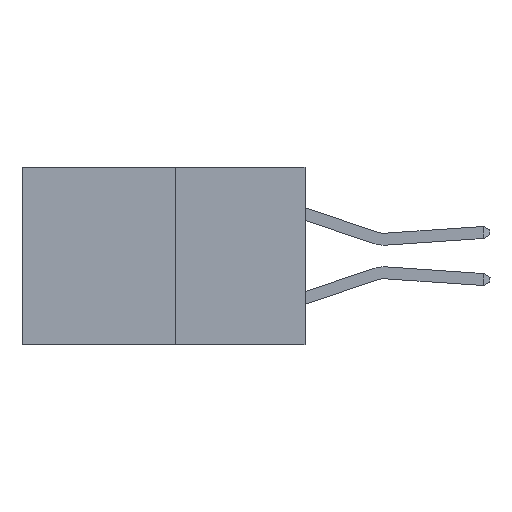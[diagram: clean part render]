
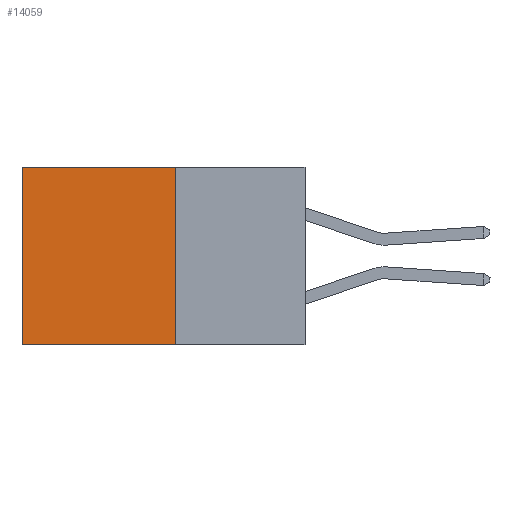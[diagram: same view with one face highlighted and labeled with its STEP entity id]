
A CAD part, left-side view. The second image highlights one B-rep face of the part: STEP entity #14059.
In plain terms, the highlighted planar face has unit normal (-1, 0, 0).
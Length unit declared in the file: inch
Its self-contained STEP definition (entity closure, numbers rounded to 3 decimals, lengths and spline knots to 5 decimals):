
#8 = DIRECTION ( 'NONE',  ( 0., 0., -1. ) ) ;
#66 = ORIENTED_EDGE ( 'NONE', *, *, #6767, .T. ) ;
#290 = VECTOR ( 'NONE', #7099, 39.37008 ) ;
#458 = CARTESIAN_POINT ( 'NONE',  ( 0.277, 0.27, 0. ) ) ;
#850 = VERTEX_POINT ( 'NONE', #9230 ) ;
#887 = VERTEX_POINT ( 'NONE', #6599 ) ;
#943 = LINE ( 'NONE', #10141, #3595 ) ;
#1780 = EDGE_CURVE ( 'NONE', #6536, #850, #3207, .T. ) ;
#3207 = LINE ( 'NONE', #3395, #6185 ) ;
#3395 = CARTESIAN_POINT ( 'NONE',  ( 0.277, 0.27, -0.37 ) ) ;
#3595 = VECTOR ( 'NONE', #10285, 39.37008 ) ;
#6132 = VECTOR ( 'NONE', #8037, 39.37008 ) ;
#6185 = VECTOR ( 'NONE', #12896, 39.37008 ) ;
#6522 = LINE ( 'NONE', #6680, #6132 ) ;
#6536 = VERTEX_POINT ( 'NONE', #458 ) ;
#6599 = CARTESIAN_POINT ( 'NONE',  ( 0.277, 0.59, -0.37 ) ) ;
#6680 = CARTESIAN_POINT ( 'NONE',  ( 0.277, 0.59, -0.37 ) ) ;
#6767 = EDGE_CURVE ( 'NONE', #6536, #9168, #943, .T. ) ;
#7096 = LINE ( 'NONE', #10864, #290 ) ;
#7099 = DIRECTION ( 'NONE',  ( 0., 1., 0. ) ) ;
#7666 = DIRECTION ( 'NONE',  ( 1., 0., 0. ) ) ;
#8037 = DIRECTION ( 'NONE',  ( 0., 0., -1. ) ) ;
#8387 = AXIS2_PLACEMENT_3D ( 'NONE', #13862, #7666, #8 ) ;
#9168 = VERTEX_POINT ( 'NONE', #11903 ) ;
#9230 = CARTESIAN_POINT ( 'NONE',  ( 0.277, 0.27, -0.37 ) ) ;
#10141 = CARTESIAN_POINT ( 'NONE',  ( 0.277, 0.27, 0. ) ) ;
#10285 = DIRECTION ( 'NONE',  ( 0., 1., 0. ) ) ;
#10406 = ORIENTED_EDGE ( 'NONE', *, *, #14451, .F. ) ;
#10864 = CARTESIAN_POINT ( 'NONE',  ( 0.277, 0.27, -0.37 ) ) ;
#11903 = CARTESIAN_POINT ( 'NONE',  ( 0.277, 0.59, 0. ) ) ;
#11928 = ORIENTED_EDGE ( 'NONE', *, *, #1780, .F. ) ;
#12613 = PLANE ( 'NONE',  #8387 ) ;
#12896 = DIRECTION ( 'NONE',  ( 0., 0., -1. ) ) ;
#13847 = EDGE_LOOP ( 'NONE', ( #14259, #10406, #11928, #66 ) ) ;
#13862 = CARTESIAN_POINT ( 'NONE',  ( 0.277, 0.27, -0.37 ) ) ;
#14059 = ADVANCED_FACE ( 'NONE', ( #15890 ), #12613, .F. ) ;
#14259 = ORIENTED_EDGE ( 'NONE', *, *, #14266, .T. ) ;
#14266 = EDGE_CURVE ( 'NONE', #9168, #887, #6522, .T. ) ;
#14451 = EDGE_CURVE ( 'NONE', #850, #887, #7096, .T. ) ;
#15890 = FACE_OUTER_BOUND ( 'NONE', #13847, .T. ) ;
